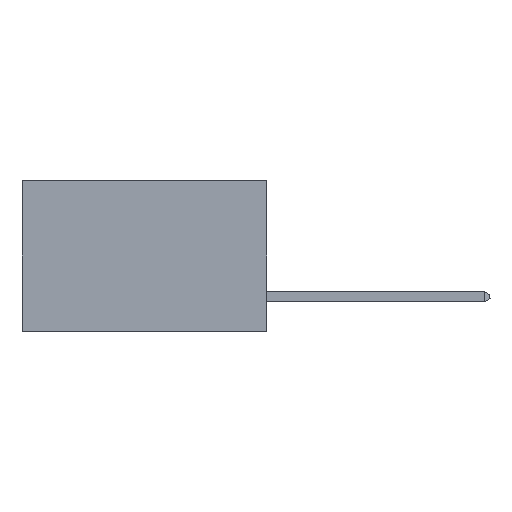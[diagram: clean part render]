
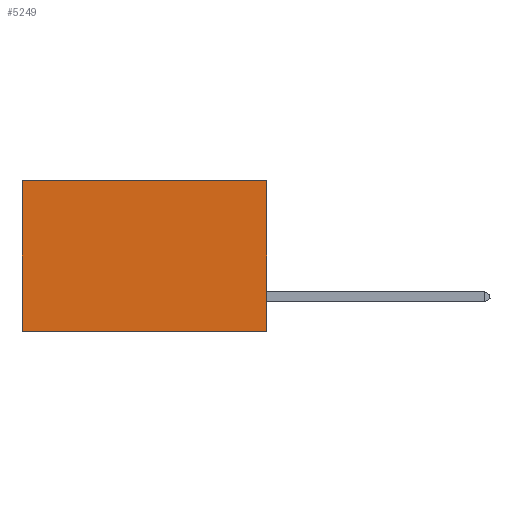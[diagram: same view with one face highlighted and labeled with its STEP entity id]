
A CAD part, left-side view. The second image highlights one B-rep face of the part: STEP entity #5249.
In plain terms, the highlighted planar face has unit normal (-1, 0, 0).
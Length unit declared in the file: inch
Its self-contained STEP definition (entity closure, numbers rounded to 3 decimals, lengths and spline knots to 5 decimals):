
#228 = CARTESIAN_POINT ( 'NONE',  ( 0.2875, 0., 0. ) ) ;
#354 = VERTEX_POINT ( 'NONE', #13648 ) ;
#691 = VECTOR ( 'NONE', #6590, 39.37008 ) ;
#1346 = ORIENTED_EDGE ( 'NONE', *, *, #9518, .F. ) ;
#1722 = DIRECTION ( 'NONE',  ( 0., 0., -1. ) ) ;
#2084 = DIRECTION ( 'NONE',  ( 1., 0., 0. ) ) ;
#3360 = VERTEX_POINT ( 'NONE', #14533 ) ;
#3462 = EDGE_CURVE ( 'NONE', #354, #3360, #14896, .T. ) ;
#3490 = CARTESIAN_POINT ( 'NONE',  ( 0.2875, 0.6, 0. ) ) ;
#3493 = LINE ( 'NONE', #7827, #15004 ) ;
#4302 = ORIENTED_EDGE ( 'NONE', *, *, #3462, .T. ) ;
#4687 = CARTESIAN_POINT ( 'NONE',  ( 0.2875, 0.6, -0.37 ) ) ;
#5249 = ADVANCED_FACE ( 'NONE', ( #11407 ), #8971, .F. ) ;
#5725 = EDGE_LOOP ( 'NONE', ( #6897, #12523, #1346, #4302 ) ) ;
#6272 = CARTESIAN_POINT ( 'NONE',  ( 0.2875, 0., -0.37 ) ) ;
#6570 = CARTESIAN_POINT ( 'NONE',  ( 0.2875, 0., 0. ) ) ;
#6590 = DIRECTION ( 'NONE',  ( 0., 1., 0. ) ) ;
#6887 = VERTEX_POINT ( 'NONE', #6272 ) ;
#6897 = ORIENTED_EDGE ( 'NONE', *, *, #7799, .T. ) ;
#7187 = DIRECTION ( 'NONE',  ( 0., 0., -1. ) ) ;
#7799 = EDGE_CURVE ( 'NONE', #3360, #15701, #12974, .T. ) ;
#7827 = CARTESIAN_POINT ( 'NONE',  ( 0.2875, 0., 0. ) ) ;
#8144 = DIRECTION ( 'NONE',  ( 0., 0., -1. ) ) ;
#8832 = AXIS2_PLACEMENT_3D ( 'NONE', #6570, #2084, #8144 ) ;
#8971 = PLANE ( 'NONE',  #8832 ) ;
#9518 = EDGE_CURVE ( 'NONE', #354, #6887, #3493, .T. ) ;
#10314 = VECTOR ( 'NONE', #12515, 39.37008 ) ;
#11407 = FACE_OUTER_BOUND ( 'NONE', #5725, .T. ) ;
#12515 = DIRECTION ( 'NONE',  ( 0., 1., 0. ) ) ;
#12523 = ORIENTED_EDGE ( 'NONE', *, *, #14231, .F. ) ;
#12658 = CARTESIAN_POINT ( 'NONE',  ( 0.2875, 0., -0.37 ) ) ;
#12974 = LINE ( 'NONE', #3490, #14859 ) ;
#13560 = LINE ( 'NONE', #12658, #691 ) ;
#13648 = CARTESIAN_POINT ( 'NONE',  ( 0.2875, 0., 0. ) ) ;
#14231 = EDGE_CURVE ( 'NONE', #6887, #15701, #13560, .T. ) ;
#14533 = CARTESIAN_POINT ( 'NONE',  ( 0.2875, 0.6, 0. ) ) ;
#14859 = VECTOR ( 'NONE', #7187, 39.37008 ) ;
#14896 = LINE ( 'NONE', #228, #10314 ) ;
#15004 = VECTOR ( 'NONE', #1722, 39.37008 ) ;
#15701 = VERTEX_POINT ( 'NONE', #4687 ) ;
